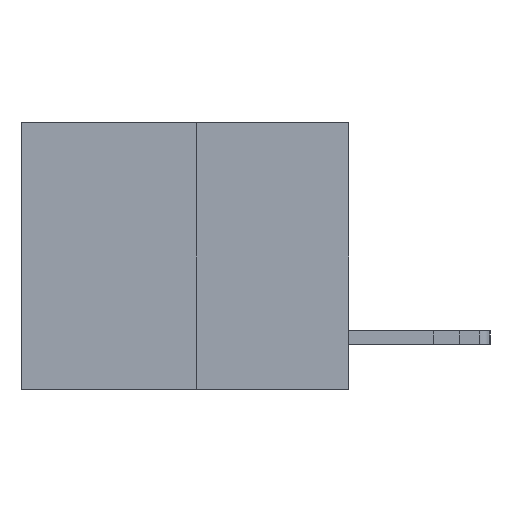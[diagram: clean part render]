
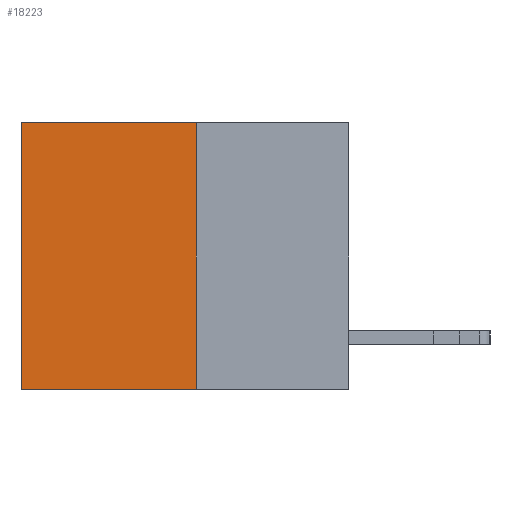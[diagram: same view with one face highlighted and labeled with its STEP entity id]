
A CAD part, left-side view. The second image highlights one B-rep face of the part: STEP entity #18223.
In plain terms, the highlighted planar face has unit normal (-1, 0, 0).
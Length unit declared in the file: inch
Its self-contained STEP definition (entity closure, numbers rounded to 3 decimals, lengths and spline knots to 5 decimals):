
#198 = CARTESIAN_POINT ( 'NONE',  ( 0.3165, 0.28, 0. ) ) ;
#280 = DIRECTION ( 'NONE',  ( 0., 0., -1. ) ) ;
#522 = CARTESIAN_POINT ( 'NONE',  ( 0.3165, 0.28, -0.49 ) ) ;
#1295 = DIRECTION ( 'NONE',  ( 0., 0., -1. ) ) ;
#1979 = LINE ( 'NONE', #12287, #11731 ) ;
#2403 = VERTEX_POINT ( 'NONE', #12919 ) ;
#2925 = LINE ( 'NONE', #8618, #7677 ) ;
#4589 = EDGE_CURVE ( 'NONE', #17012, #16679, #2925, .T. ) ;
#4764 = DIRECTION ( 'NONE',  ( 1., 0., 0. ) ) ;
#5105 = AXIS2_PLACEMENT_3D ( 'NONE', #11322, #4764, #1295 ) ;
#5632 = EDGE_CURVE ( 'NONE', #17012, #2403, #20180, .T. ) ;
#7677 = VECTOR ( 'NONE', #280, 39.37008 ) ;
#7949 = ORIENTED_EDGE ( 'NONE', *, *, #4589, .F. ) ;
#8072 = PLANE ( 'NONE',  #5105 ) ;
#8618 = CARTESIAN_POINT ( 'NONE',  ( 0.3165, 0.28, -0.49 ) ) ;
#10283 = ORIENTED_EDGE ( 'NONE', *, *, #5632, .T. ) ;
#10690 = DIRECTION ( 'NONE',  ( 0., 0., -1. ) ) ;
#10844 = CARTESIAN_POINT ( 'NONE',  ( 0.3165, 0.28, 0. ) ) ;
#11322 = CARTESIAN_POINT ( 'NONE',  ( 0.3165, 0.28, -0.49 ) ) ;
#11658 = ORIENTED_EDGE ( 'NONE', *, *, #14901, .T. ) ;
#11731 = VECTOR ( 'NONE', #10690, 39.37008 ) ;
#11940 = EDGE_LOOP ( 'NONE', ( #11658, #16893, #7949, #10283 ) ) ;
#12098 = VECTOR ( 'NONE', #18182, 39.37008 ) ;
#12215 = EDGE_CURVE ( 'NONE', #16679, #17040, #19941, .T. ) ;
#12287 = CARTESIAN_POINT ( 'NONE',  ( 0.3165, 0.6, -0.49 ) ) ;
#12919 = CARTESIAN_POINT ( 'NONE',  ( 0.3165, 0.6, 0. ) ) ;
#12946 = CARTESIAN_POINT ( 'NONE',  ( 0.3165, 0.6, -0.49 ) ) ;
#13526 = FACE_OUTER_BOUND ( 'NONE', #11940, .T. ) ;
#14168 = DIRECTION ( 'NONE',  ( 0., 1., 0. ) ) ;
#14901 = EDGE_CURVE ( 'NONE', #2403, #17040, #1979, .T. ) ;
#16679 = VERTEX_POINT ( 'NONE', #522 ) ;
#16893 = ORIENTED_EDGE ( 'NONE', *, *, #12215, .F. ) ;
#17012 = VERTEX_POINT ( 'NONE', #198 ) ;
#17040 = VERTEX_POINT ( 'NONE', #12946 ) ;
#18182 = DIRECTION ( 'NONE',  ( 0., 1., 0. ) ) ;
#18223 = ADVANCED_FACE ( 'NONE', ( #13526 ), #8072, .F. ) ;
#19123 = VECTOR ( 'NONE', #14168, 39.37008 ) ;
#19941 = LINE ( 'NONE', #21368, #12098 ) ;
#20180 = LINE ( 'NONE', #10844, #19123 ) ;
#21368 = CARTESIAN_POINT ( 'NONE',  ( 0.3165, 0.28, -0.49 ) ) ;
